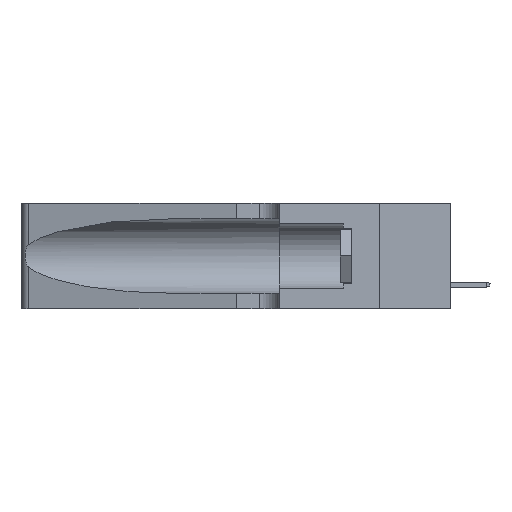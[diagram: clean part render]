
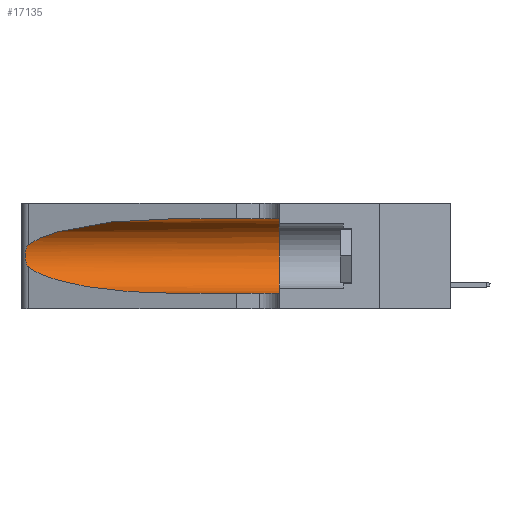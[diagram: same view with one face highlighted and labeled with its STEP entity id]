
A CAD part, left-side view. The second image highlights one B-rep face of the part: STEP entity #17135.
In plain terms, the highlighted cylindrical face has radius 3.308 mm (diameter 6.617 mm), a partial arc.
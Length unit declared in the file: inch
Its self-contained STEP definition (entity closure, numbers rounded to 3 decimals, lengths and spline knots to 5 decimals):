
#112 = CARTESIAN_POINT ( 'NONE',  ( 0.25487, 1.22718, 0.14631 ) ) ;
#655 = CARTESIAN_POINT ( 'NONE',  ( 0.26075, 1.23896, 0.178 ) ) ;
#1189 = B_SPLINE_CURVE_WITH_KNOTS ( 'NONE', 3,
 ( #6283, #24714, #15794, #15409, #36402, #27191, #9927, #655, #9552, #30236, #6101, #21387, #6666, #18495 ),
 .UNSPECIFIED., .F., .F.,
 ( 4, 2, 2, 2, 2, 2, 4 ),
 ( 0., 0.00027, 0.00053, 0.00107, 0.0016, 0.00187, 0.00214 ),
 .UNSPECIFIED. ) ;
#1943 = CARTESIAN_POINT ( 'NONE',  ( 0.1305, 0.35, 0.31525 ) ) ;
#2081 = CARTESIAN_POINT ( 'NONE',  ( 0.25487, 1.22718, 0.14631 ) ) ;
#3413 = CARTESIAN_POINT ( 'NONE',  ( 0.1305, 0.72297, 0.05475 ) ) ;
#4788 = CARTESIAN_POINT ( 'NONE',  ( 0.1305, 1.61858, 0.05475 ) ) ;
#5236 = VERTEX_POINT ( 'NONE', #30221 ) ;
#6101 = CARTESIAN_POINT ( 'NONE',  ( 0.25789, 1.23486, 0.15765 ) ) ;
#6253 = CARTESIAN_POINT ( 'NONE',  ( 0.25487, 1.22718, 0.22369 ) ) ;
#6283 = CARTESIAN_POINT ( 'NONE',  ( 0.25487, 1.22718, 0.22369 ) ) ;
#6666 = CARTESIAN_POINT ( 'NONE',  ( 0.25555, 1.22993, 0.14849 ) ) ;
#7995 =( BOUNDED_CURVE ( )  B_SPLINE_CURVE ( 3, ( #112, #15042, #26631, #3413 ),
 .UNSPECIFIED., .F., .F. ) 
 B_SPLINE_CURVE_WITH_KNOTS ( ( 4, 4 ),
 ( 3.44316, 4.71239 ),
 .UNSPECIFIED. ) 
 CURVE ( )  GEOMETRIC_REPRESENTATION_ITEM ( )  RATIONAL_B_SPLINE_CURVE ( ( 1., 0.87, 0.87, 1. ) ) 
 REPRESENTATION_ITEM ( '' )  );
#8855 = EDGE_CURVE ( 'NONE', #9102, #13068, #11531, .T. ) ;
#8961 = CARTESIAN_POINT ( 'NONE',  ( 0.1305, 0.72297, 0.31525 ) ) ;
#9102 = VERTEX_POINT ( 'NONE', #32789 ) ;
#9128 = LINE ( 'NONE', #23505, #31754 ) ;
#9515 =( BOUNDED_CURVE ( )  B_SPLINE_CURVE ( 3, ( #8961, #11891, #23902, #6253 ),
 .UNSPECIFIED., .F., .T. ) 
 B_SPLINE_CURVE_WITH_KNOTS ( ( 4, 4 ),
 ( 1.5708, 2.84003 ),
 .UNSPECIFIED. ) 
 CURVE ( )  GEOMETRIC_REPRESENTATION_ITEM ( )  RATIONAL_B_SPLINE_CURVE ( ( 1., 0.87, 0.87, 1. ) ) 
 REPRESENTATION_ITEM ( '' )  );
#9552 = CARTESIAN_POINT ( 'NONE',  ( 0.26017, 1.23833, 0.17102 ) ) ;
#9927 = CARTESIAN_POINT ( 'NONE',  ( 0.26075, 1.23896, 0.19203 ) ) ;
#10585 = EDGE_LOOP ( 'NONE', ( #22876, #18626, #31691, #12090, #11828, #37044 ) ) ;
#10979 = EDGE_CURVE ( 'NONE', #23221, #19753, #1189, .T. ) ;
#11100 = CARTESIAN_POINT ( 'NONE',  ( 0.1305, 0.35, 0.05475 ) ) ;
#11253 = DIRECTION ( 'NONE',  ( 0., 0., -1. ) ) ;
#11531 = LINE ( 'NONE', #4788, #15306 ) ;
#11828 = ORIENTED_EDGE ( 'NONE', *, *, #29081, .F. ) ;
#11891 = CARTESIAN_POINT ( 'NONE',  ( 0.18966, 0.96281, 0.31525 ) ) ;
#12090 = ORIENTED_EDGE ( 'NONE', *, *, #8855, .T. ) ;
#13068 = VERTEX_POINT ( 'NONE', #11100 ) ;
#13714 = EDGE_CURVE ( 'NONE', #5236, #18929, #9128, .T. ) ;
#13994 = FACE_OUTER_BOUND ( 'NONE', #10585, .T. ) ;
#14496 = DIRECTION ( 'NONE',  ( 0., 0., 1. ) ) ;
#15042 = CARTESIAN_POINT ( 'NONE',  ( 0.2373, 1.15595, 0.08982 ) ) ;
#15306 = VECTOR ( 'NONE', #16623, 39.37008 ) ;
#15409 = CARTESIAN_POINT ( 'NONE',  ( 0.25787, 1.23484, 0.2124 ) ) ;
#15794 = CARTESIAN_POINT ( 'NONE',  ( 0.25639, 1.23184, 0.21858 ) ) ;
#16623 = DIRECTION ( 'NONE',  ( 0., -1., 0. ) ) ;
#17135 = ADVANCED_FACE ( 'NONE', ( #13994 ), #22919, .F. ) ;
#17280 = DIRECTION ( 'NONE',  ( 0., -1., 0. ) ) ;
#18495 = CARTESIAN_POINT ( 'NONE',  ( 0.25487, 1.22718, 0.14631 ) ) ;
#18510 = CARTESIAN_POINT ( 'NONE',  ( 0.25487, 1.22718, 0.22369 ) ) ;
#18626 = ORIENTED_EDGE ( 'NONE', *, *, #10979, .T. ) ;
#18762 = AXIS2_PLACEMENT_3D ( 'NONE', #31681, #37484, #14496 ) ;
#18929 = VERTEX_POINT ( 'NONE', #1943 ) ;
#19753 = VERTEX_POINT ( 'NONE', #2081 ) ;
#21387 = CARTESIAN_POINT ( 'NONE',  ( 0.25639, 1.23186, 0.15144 ) ) ;
#22876 = ORIENTED_EDGE ( 'NONE', *, *, #36409, .T. ) ;
#22919 = CYLINDRICAL_SURFACE ( 'NONE', #24542, 0.13025 ) ;
#23221 = VERTEX_POINT ( 'NONE', #18510 ) ;
#23298 = CARTESIAN_POINT ( 'NONE',  ( 0.1305, 1.61858, 0.185 ) ) ;
#23505 = CARTESIAN_POINT ( 'NONE',  ( 0.1305, 1.61858, 0.31525 ) ) ;
#23902 = CARTESIAN_POINT ( 'NONE',  ( 0.2373, 1.15595, 0.28018 ) ) ;
#24542 = AXIS2_PLACEMENT_3D ( 'NONE', #23298, #17280, #11253 ) ;
#24714 = CARTESIAN_POINT ( 'NONE',  ( 0.25555, 1.22994, 0.2215 ) ) ;
#26631 = CARTESIAN_POINT ( 'NONE',  ( 0.18966, 0.96281, 0.05475 ) ) ;
#27191 = CARTESIAN_POINT ( 'NONE',  ( 0.26018, 1.23835, 0.19895 ) ) ;
#29081 = EDGE_CURVE ( 'NONE', #18929, #13068, #37241, .T. ) ;
#30221 = CARTESIAN_POINT ( 'NONE',  ( 0.1305, 0.72297, 0.31525 ) ) ;
#30236 = CARTESIAN_POINT ( 'NONE',  ( 0.25856, 1.23593, 0.16098 ) ) ;
#31681 = CARTESIAN_POINT ( 'NONE',  ( 0.1305, 0.35, 0.185 ) ) ;
#31691 = ORIENTED_EDGE ( 'NONE', *, *, #35041, .T. ) ;
#31754 = VECTOR ( 'NONE', #35972, 39.37008 ) ;
#32789 = CARTESIAN_POINT ( 'NONE',  ( 0.1305, 0.72297, 0.05475 ) ) ;
#35041 = EDGE_CURVE ( 'NONE', #19753, #9102, #7995, .T. ) ;
#35972 = DIRECTION ( 'NONE',  ( 0., -1., 0. ) ) ;
#36402 = CARTESIAN_POINT ( 'NONE',  ( 0.25854, 1.2359, 0.20912 ) ) ;
#36409 = EDGE_CURVE ( 'NONE', #5236, #23221, #9515, .T. ) ;
#37044 = ORIENTED_EDGE ( 'NONE', *, *, #13714, .F. ) ;
#37241 = CIRCLE ( 'NONE', #18762, 0.13025 ) ;
#37484 = DIRECTION ( 'NONE',  ( 0., 1., 0. ) ) ;
